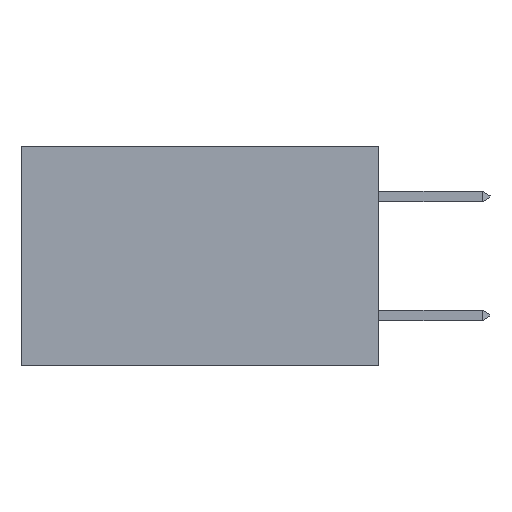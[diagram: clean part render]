
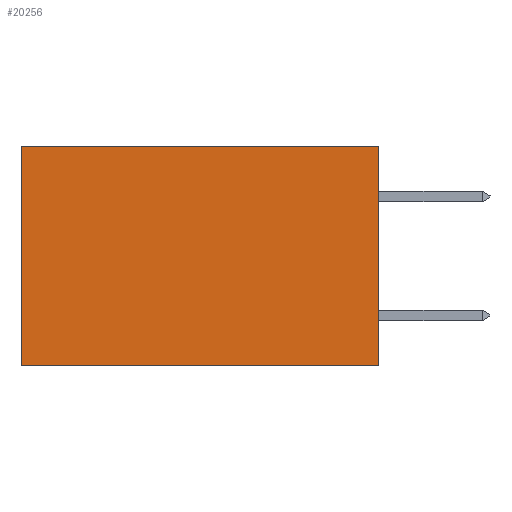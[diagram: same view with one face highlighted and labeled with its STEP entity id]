
A CAD part, left-side view. The second image highlights one B-rep face of the part: STEP entity #20256.
In plain terms, the highlighted planar face has unit normal (-1, 0, 0).
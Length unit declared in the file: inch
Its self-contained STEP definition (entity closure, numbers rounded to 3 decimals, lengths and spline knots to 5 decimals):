
#409 = CARTESIAN_POINT ( 'NONE',  ( 0.2615, 0.6, -0.37 ) ) ;
#1574 = VERTEX_POINT ( 'NONE', #409 ) ;
#4242 = DIRECTION ( 'NONE',  ( 0., 1., 0. ) ) ;
#4320 = EDGE_CURVE ( 'NONE', #9393, #16521, #17023, .T. ) ;
#4837 = FACE_OUTER_BOUND ( 'NONE', #22779, .T. ) ;
#6312 = CARTESIAN_POINT ( 'NONE',  ( 0.2615, 0., -0.37 ) ) ;
#6343 = CARTESIAN_POINT ( 'NONE',  ( 0.2615, 0., 0. ) ) ;
#8136 = CARTESIAN_POINT ( 'NONE',  ( 0.2615, 0., -0.37 ) ) ;
#8984 = DIRECTION ( 'NONE',  ( 1., 0., 0. ) ) ;
#9075 = LINE ( 'NONE', #17570, #11039 ) ;
#9393 = VERTEX_POINT ( 'NONE', #14067 ) ;
#10005 = VECTOR ( 'NONE', #4242, 39.37008 ) ;
#10123 = VECTOR ( 'NONE', #20688, 39.37008 ) ;
#10760 = ORIENTED_EDGE ( 'NONE', *, *, #4320, .F. ) ;
#11039 = VECTOR ( 'NONE', #19661, 39.37008 ) ;
#11477 = CARTESIAN_POINT ( 'NONE',  ( 0.2615, 0., -0.37 ) ) ;
#12743 = ORIENTED_EDGE ( 'NONE', *, *, #21295, .F. ) ;
#14067 = CARTESIAN_POINT ( 'NONE',  ( 0.2615, 0., 0. ) ) ;
#15642 = DIRECTION ( 'NONE',  ( 0., 0., -1. ) ) ;
#16521 = VERTEX_POINT ( 'NONE', #11477 ) ;
#16619 = DIRECTION ( 'NONE',  ( 0., 0., -1. ) ) ;
#16753 = LINE ( 'NONE', #6312, #10005 ) ;
#17023 = LINE ( 'NONE', #8136, #27265 ) ;
#17090 = AXIS2_PLACEMENT_3D ( 'NONE', #26239, #8984, #15642 ) ;
#17259 = ORIENTED_EDGE ( 'NONE', *, *, #27032, .T. ) ;
#17570 = CARTESIAN_POINT ( 'NONE',  ( 0.2615, 0.6, -0.37 ) ) ;
#19661 = DIRECTION ( 'NONE',  ( 0., 0., -1. ) ) ;
#20256 = ADVANCED_FACE ( 'NONE', ( #4837 ), #26098, .F. ) ;
#20688 = DIRECTION ( 'NONE',  ( 0., 1., 0. ) ) ;
#20894 = VERTEX_POINT ( 'NONE', #24887 ) ;
#21295 = EDGE_CURVE ( 'NONE', #16521, #1574, #16753, .T. ) ;
#22498 = ORIENTED_EDGE ( 'NONE', *, *, #26259, .T. ) ;
#22779 = EDGE_LOOP ( 'NONE', ( #17259, #12743, #10760, #22498 ) ) ;
#24887 = CARTESIAN_POINT ( 'NONE',  ( 0.2615, 0.6, 0. ) ) ;
#26098 = PLANE ( 'NONE',  #17090 ) ;
#26239 = CARTESIAN_POINT ( 'NONE',  ( 0.2615, 0., -0.37 ) ) ;
#26259 = EDGE_CURVE ( 'NONE', #9393, #20894, #27208, .T. ) ;
#27032 = EDGE_CURVE ( 'NONE', #20894, #1574, #9075, .T. ) ;
#27208 = LINE ( 'NONE', #6343, #10123 ) ;
#27265 = VECTOR ( 'NONE', #16619, 39.37008 ) ;
